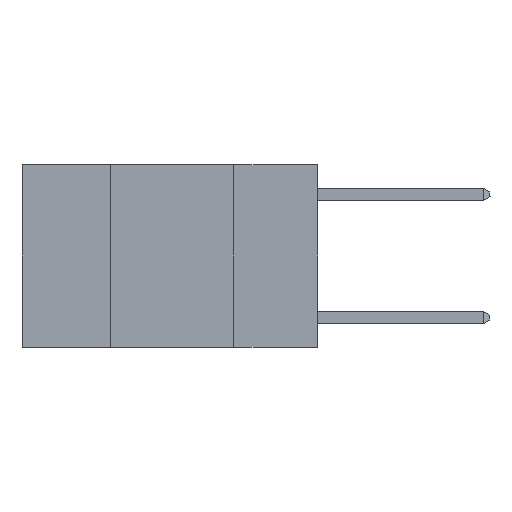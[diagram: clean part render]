
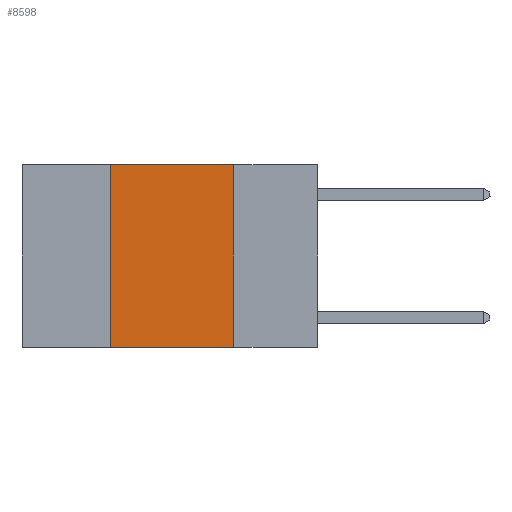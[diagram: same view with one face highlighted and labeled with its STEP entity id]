
A CAD part, left-side view. The second image highlights one B-rep face of the part: STEP entity #8598.
In plain terms, the highlighted planar face has unit normal (-1, 0, 0).
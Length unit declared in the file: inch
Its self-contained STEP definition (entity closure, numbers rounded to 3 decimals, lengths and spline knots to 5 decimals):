
#1022 = VERTEX_POINT ( 'NONE', #8067 ) ;
#2216 = EDGE_LOOP ( 'NONE', ( #14705, #5917, #11973, #15059 ) ) ;
#2437 = EDGE_CURVE ( 'NONE', #4049, #10847, #2853, .T. ) ;
#2458 = VECTOR ( 'NONE', #5426, 39.37008 ) ;
#2853 = LINE ( 'NONE', #5089, #2458 ) ;
#3254 = CARTESIAN_POINT ( 'NONE',  ( 0., 0.17, -0.37 ) ) ;
#4032 = PLANE ( 'NONE',  #10181 ) ;
#4049 = VERTEX_POINT ( 'NONE', #4284 ) ;
#4057 = VECTOR ( 'NONE', #12034, 39.37008 ) ;
#4284 = CARTESIAN_POINT ( 'NONE',  ( 0., 0.17, 0. ) ) ;
#4442 = VECTOR ( 'NONE', #13134, 39.37008 ) ;
#4461 = DIRECTION ( 'NONE',  ( 0., 0., 1. ) ) ;
#5089 = CARTESIAN_POINT ( 'NONE',  ( 0., 0.17, 0. ) ) ;
#5228 = DIRECTION ( 'NONE',  ( 0., 0., -1. ) ) ;
#5426 = DIRECTION ( 'NONE',  ( 0., 0., -1. ) ) ;
#5917 = ORIENTED_EDGE ( 'NONE', *, *, #10538, .F. ) ;
#7528 = LINE ( 'NONE', #8646, #4057 ) ;
#8067 = CARTESIAN_POINT ( 'NONE',  ( 0., 0.42, 0. ) ) ;
#8598 = ADVANCED_FACE ( 'NONE', ( #9924 ), #4032, .F. ) ;
#8646 = CARTESIAN_POINT ( 'NONE',  ( 0., 0.6, -0.37 ) ) ;
#9029 = VECTOR ( 'NONE', #4461, 39.37008 ) ;
#9034 = CARTESIAN_POINT ( 'NONE',  ( 0., 0.42, -0.37 ) ) ;
#9838 = CARTESIAN_POINT ( 'NONE',  ( 0., 0.6, 0. ) ) ;
#9917 = EDGE_CURVE ( 'NONE', #14488, #10847, #7528, .T. ) ;
#9924 = FACE_OUTER_BOUND ( 'NONE', #2216, .T. ) ;
#10181 = AXIS2_PLACEMENT_3D ( 'NONE', #9838, #12072, #5228 ) ;
#10538 = EDGE_CURVE ( 'NONE', #1022, #4049, #10603, .T. ) ;
#10603 = LINE ( 'NONE', #11982, #4442 ) ;
#10847 = VERTEX_POINT ( 'NONE', #3254 ) ;
#11471 = CARTESIAN_POINT ( 'NONE',  ( 0., 0.42, 0. ) ) ;
#11973 = ORIENTED_EDGE ( 'NONE', *, *, #12539, .F. ) ;
#11982 = CARTESIAN_POINT ( 'NONE',  ( 0., 0.6, 0. ) ) ;
#12034 = DIRECTION ( 'NONE',  ( 0., -1., 0. ) ) ;
#12072 = DIRECTION ( 'NONE',  ( 1., 0., 0. ) ) ;
#12539 = EDGE_CURVE ( 'NONE', #14488, #1022, #15101, .T. ) ;
#13134 = DIRECTION ( 'NONE',  ( 0., -1., 0. ) ) ;
#14488 = VERTEX_POINT ( 'NONE', #9034 ) ;
#14705 = ORIENTED_EDGE ( 'NONE', *, *, #2437, .F. ) ;
#15059 = ORIENTED_EDGE ( 'NONE', *, *, #9917, .T. ) ;
#15101 = LINE ( 'NONE', #11471, #9029 ) ;
